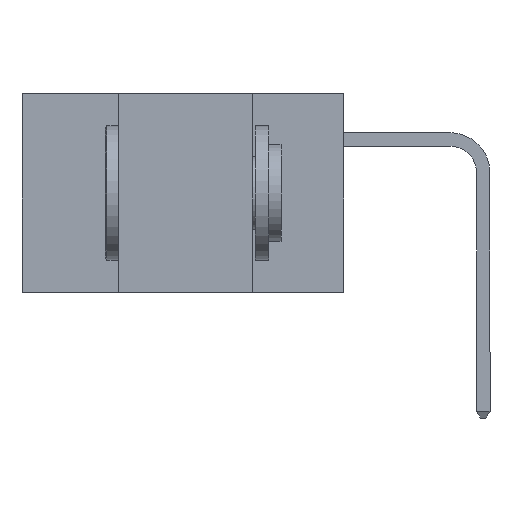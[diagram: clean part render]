
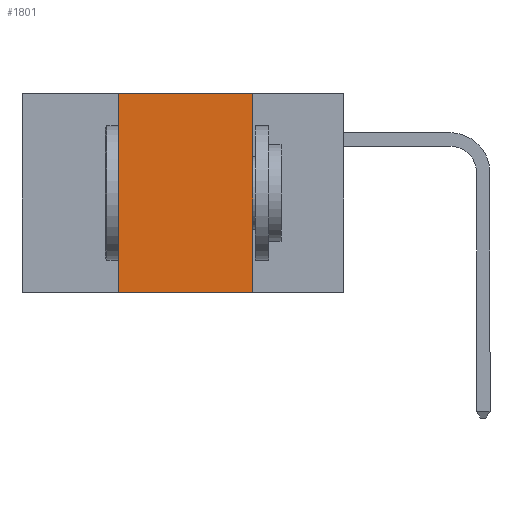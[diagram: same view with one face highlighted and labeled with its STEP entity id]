
A CAD part, left-side view. The second image highlights one B-rep face of the part: STEP entity #1801.
In plain terms, the highlighted planar face has unit normal (-1, 0, 0).
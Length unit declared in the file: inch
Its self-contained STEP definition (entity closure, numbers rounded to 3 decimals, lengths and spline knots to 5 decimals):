
#681 = LINE ( 'NONE', #17478, #4863 ) ;
#1221 = AXIS2_PLACEMENT_3D ( 'NONE', #22617, #5709, #5683 ) ;
#1801 = ADVANCED_FACE ( 'NONE', ( #12442 ), #18911, .F. ) ;
#4466 = ORIENTED_EDGE ( 'NONE', *, *, #4604, .F. ) ;
#4604 = EDGE_CURVE ( 'NONE', #16446, #19083, #20460, .T. ) ;
#4863 = VECTOR ( 'NONE', #10520, 39.37008 ) ;
#5683 = DIRECTION ( 'NONE',  ( 0., 0., -1. ) ) ;
#5709 = DIRECTION ( 'NONE',  ( 1., 0., 0. ) ) ;
#6331 = CARTESIAN_POINT ( 'NONE',  ( 0., 0.42, 0. ) ) ;
#6802 = VECTOR ( 'NONE', #8522, 39.37008 ) ;
#7617 = ORIENTED_EDGE ( 'NONE', *, *, #21123, .F. ) ;
#7933 = CARTESIAN_POINT ( 'NONE',  ( 0., 0.42, 0. ) ) ;
#8522 = DIRECTION ( 'NONE',  ( 0., -1., 0. ) ) ;
#9838 = ORIENTED_EDGE ( 'NONE', *, *, #22733, .T. ) ;
#10520 = DIRECTION ( 'NONE',  ( 0., 0., -1. ) ) ;
#11540 = CARTESIAN_POINT ( 'NONE',  ( 0., 0.42, -0.37 ) ) ;
#12345 = VECTOR ( 'NONE', #16331, 39.37008 ) ;
#12442 = FACE_OUTER_BOUND ( 'NONE', #18092, .T. ) ;
#13403 = VERTEX_POINT ( 'NONE', #17777 ) ;
#13407 = CARTESIAN_POINT ( 'NONE',  ( 0., 0.17, 0. ) ) ;
#15871 = VECTOR ( 'NONE', #19574, 39.37008 ) ;
#16165 = LINE ( 'NONE', #20652, #6802 ) ;
#16331 = DIRECTION ( 'NONE',  ( 0., 0., 1. ) ) ;
#16446 = VERTEX_POINT ( 'NONE', #11540 ) ;
#17428 = ORIENTED_EDGE ( 'NONE', *, *, #22504, .F. ) ;
#17478 = CARTESIAN_POINT ( 'NONE',  ( 0., 0.17, 0. ) ) ;
#17777 = CARTESIAN_POINT ( 'NONE',  ( 0., 0.17, -0.37 ) ) ;
#18092 = EDGE_LOOP ( 'NONE', ( #7617, #17428, #4466, #9838 ) ) ;
#18911 = PLANE ( 'NONE',  #1221 ) ;
#19083 = VERTEX_POINT ( 'NONE', #6331 ) ;
#19574 = DIRECTION ( 'NONE',  ( 0., -1., 0. ) ) ;
#20460 = LINE ( 'NONE', #7933, #12345 ) ;
#20478 = LINE ( 'NONE', #21260, #15871 ) ;
#20652 = CARTESIAN_POINT ( 'NONE',  ( 0., 0.6, 0. ) ) ;
#21123 = EDGE_CURVE ( 'NONE', #22360, #13403, #681, .T. ) ;
#21260 = CARTESIAN_POINT ( 'NONE',  ( 0., 0.6, -0.37 ) ) ;
#22360 = VERTEX_POINT ( 'NONE', #13407 ) ;
#22504 = EDGE_CURVE ( 'NONE', #19083, #22360, #16165, .T. ) ;
#22617 = CARTESIAN_POINT ( 'NONE',  ( 0., 0.6, 0. ) ) ;
#22733 = EDGE_CURVE ( 'NONE', #16446, #13403, #20478, .T. ) ;
